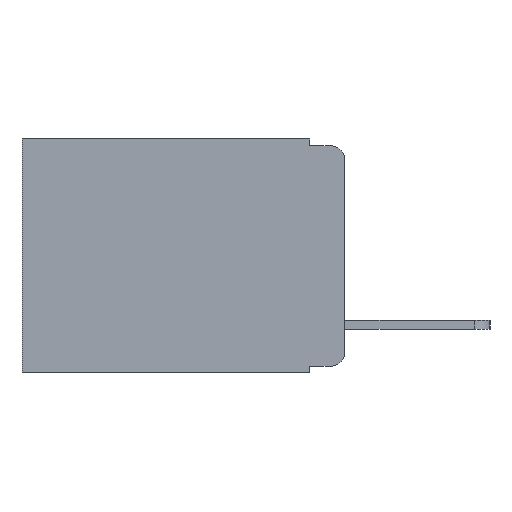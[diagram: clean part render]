
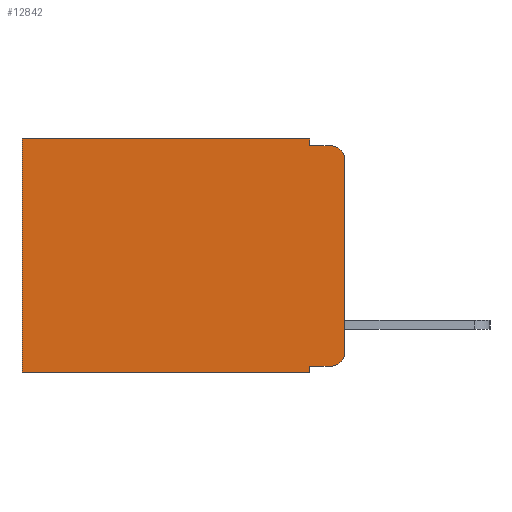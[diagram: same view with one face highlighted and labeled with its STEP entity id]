
A CAD part, left-side view. The second image highlights one B-rep face of the part: STEP entity #12842.
In plain terms, the highlighted planar face has unit normal (-1, 0, 0).
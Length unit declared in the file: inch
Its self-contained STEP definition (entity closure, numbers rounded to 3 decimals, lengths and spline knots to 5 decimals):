
#23 = CARTESIAN_POINT ( 'NONE',  ( 0.298, 0., -0.343 ) ) ;
#253 = FACE_OUTER_BOUND ( 'NONE', #6634, .T. ) ;
#566 = CARTESIAN_POINT ( 'NONE',  ( 0.298, 0.473, -0.343 ) ) ;
#773 = CARTESIAN_POINT ( 'NONE',  ( 0.298, 0., 0. ) ) ;
#2109 = DIRECTION ( 'NONE',  ( 0., 0., -1. ) ) ;
#2721 = DIRECTION ( 'NONE',  ( 0., 0., -1. ) ) ;
#2729 = VECTOR ( 'NONE', #3290, 39.37008 ) ;
#2751 = DIRECTION ( 'NONE',  ( 1., 0., 0. ) ) ;
#2919 = PLANE ( 'NONE',  #11009 ) ;
#2957 = EDGE_CURVE ( 'NONE', #6849, #13569, #20845, .T. ) ;
#3178 = ORIENTED_EDGE ( 'NONE', *, *, #3930, .F. ) ;
#3290 = DIRECTION ( 'NONE',  ( 0., 1., 0. ) ) ;
#3343 = EDGE_CURVE ( 'NONE', #10902, #22206, #21601, .T. ) ;
#3394 = CARTESIAN_POINT ( 'NONE',  ( 0.298, 0., 0. ) ) ;
#3669 = CARTESIAN_POINT ( 'NONE',  ( 0.298, 0.051, 0. ) ) ;
#3746 = DIRECTION ( 'NONE',  ( -1., 0., 0. ) ) ;
#3930 = EDGE_CURVE ( 'NONE', #8785, #4069, #19260, .T. ) ;
#3998 = EDGE_CURVE ( 'NONE', #8785, #4274, #18202, .T. ) ;
#4004 = EDGE_CURVE ( 'NONE', #4365, #4274, #5321, .T. ) ;
#4069 = VERTEX_POINT ( 'NONE', #11962 ) ;
#4159 = EDGE_CURVE ( 'NONE', #6849, #4365, #20669, .T. ) ;
#4177 = AXIS2_PLACEMENT_3D ( 'NONE', #6455, #3746, #4503 ) ;
#4274 = VERTEX_POINT ( 'NONE', #15161 ) ;
#4365 = VERTEX_POINT ( 'NONE', #20684 ) ;
#4404 = EDGE_CURVE ( 'NONE', #13569, #22206, #4499, .T. ) ;
#4458 = AXIS2_PLACEMENT_3D ( 'NONE', #13335, #13326, #20625 ) ;
#4499 = LINE ( 'NONE', #21514, #14571 ) ;
#4503 = DIRECTION ( 'NONE',  ( 0., 0., -1. ) ) ;
#4566 = EDGE_CURVE ( 'NONE', #13353, #10902, #12399, .T. ) ;
#4593 = EDGE_CURVE ( 'NONE', #13353, #18281, #21423, .T. ) ;
#4640 = EDGE_CURVE ( 'NONE', #18281, #4069, #10439, .T. ) ;
#5321 = LINE ( 'NONE', #13566, #22160 ) ;
#6455 = CARTESIAN_POINT ( 'NONE',  ( 0.298, 0.02, -0.313 ) ) ;
#6634 = EDGE_LOOP ( 'NONE', ( #3178, #12258, #16796, #21736, #22226, #18276, #18798, #11050, #15496, #20471 ) ) ;
#6849 = VERTEX_POINT ( 'NONE', #9258 ) ;
#7624 = CARTESIAN_POINT ( 'NONE',  ( 0.298, 0.02, -0.333 ) ) ;
#8089 = DIRECTION ( 'NONE',  ( 0., 1., 0. ) ) ;
#8785 = VERTEX_POINT ( 'NONE', #14760 ) ;
#8985 = CARTESIAN_POINT ( 'NONE',  ( 0.298, 0.051, -0.343 ) ) ;
#9171 = DIRECTION ( 'NONE',  ( 0., 0., -1. ) ) ;
#9258 = CARTESIAN_POINT ( 'NONE',  ( 0.298, 0.051, 0. ) ) ;
#10328 = CARTESIAN_POINT ( 'NONE',  ( 0.298, 0.473, 0. ) ) ;
#10439 = CIRCLE ( 'NONE', #4177, 0.02 ) ;
#10902 = VERTEX_POINT ( 'NONE', #8985 ) ;
#11009 = AXIS2_PLACEMENT_3D ( 'NONE', #3394, #2751, #2721 ) ;
#11050 = ORIENTED_EDGE ( 'NONE', *, *, #4566, .F. ) ;
#11850 = CARTESIAN_POINT ( 'NONE',  ( 0.298, 0., 0. ) ) ;
#11947 = DIRECTION ( 'NONE',  ( 0., 0., -1. ) ) ;
#11962 = CARTESIAN_POINT ( 'NONE',  ( 0.298, 0., -0.313 ) ) ;
#11963 = VECTOR ( 'NONE', #11977, 39.37008 ) ;
#11977 = DIRECTION ( 'NONE',  ( 0., -1., 0. ) ) ;
#12120 = DIRECTION ( 'NONE',  ( 0., 0., -1. ) ) ;
#12258 = ORIENTED_EDGE ( 'NONE', *, *, #3998, .T. ) ;
#12399 = LINE ( 'NONE', #19084, #16445 ) ;
#12842 = ADVANCED_FACE ( 'NONE', ( #253 ), #2919, .F. ) ;
#13326 = DIRECTION ( 'NONE',  ( -1., 0., 0. ) ) ;
#13335 = CARTESIAN_POINT ( 'NONE',  ( 0.298, 0.02, -0.03 ) ) ;
#13353 = VERTEX_POINT ( 'NONE', #15370 ) ;
#13379 = DIRECTION ( 'NONE',  ( 0., -1., 0. ) ) ;
#13566 = CARTESIAN_POINT ( 'NONE',  ( 0.298, 0.051, -0.01 ) ) ;
#13569 = VERTEX_POINT ( 'NONE', #10328 ) ;
#14571 = VECTOR ( 'NONE', #9171, 39.37008 ) ;
#14760 = CARTESIAN_POINT ( 'NONE',  ( 0.298, 0., -0.03 ) ) ;
#15161 = CARTESIAN_POINT ( 'NONE',  ( 0.298, 0.02, -0.01 ) ) ;
#15370 = CARTESIAN_POINT ( 'NONE',  ( 0.298, 0.051, -0.333 ) ) ;
#15429 = VECTOR ( 'NONE', #12120, 39.37008 ) ;
#15496 = ORIENTED_EDGE ( 'NONE', *, *, #4593, .T. ) ;
#15671 = VECTOR ( 'NONE', #2109, 39.37008 ) ;
#16120 = VECTOR ( 'NONE', #8089, 39.37008 ) ;
#16445 = VECTOR ( 'NONE', #11947, 39.37008 ) ;
#16796 = ORIENTED_EDGE ( 'NONE', *, *, #4004, .F. ) ;
#17062 = CARTESIAN_POINT ( 'NONE',  ( 0.298, 0.051, -0.333 ) ) ;
#18202 = CIRCLE ( 'NONE', #4458, 0.02 ) ;
#18276 = ORIENTED_EDGE ( 'NONE', *, *, #4404, .T. ) ;
#18281 = VERTEX_POINT ( 'NONE', #7624 ) ;
#18798 = ORIENTED_EDGE ( 'NONE', *, *, #3343, .F. ) ;
#19084 = CARTESIAN_POINT ( 'NONE',  ( 0.298, 0.051, 0. ) ) ;
#19260 = LINE ( 'NONE', #11850, #15429 ) ;
#20471 = ORIENTED_EDGE ( 'NONE', *, *, #4640, .T. ) ;
#20625 = DIRECTION ( 'NONE',  ( 0., 0., -1. ) ) ;
#20669 = LINE ( 'NONE', #3669, #15671 ) ;
#20684 = CARTESIAN_POINT ( 'NONE',  ( 0.298, 0.051, -0.01 ) ) ;
#20845 = LINE ( 'NONE', #773, #2729 ) ;
#21423 = LINE ( 'NONE', #17062, #11963 ) ;
#21514 = CARTESIAN_POINT ( 'NONE',  ( 0.298, 0.473, 0. ) ) ;
#21601 = LINE ( 'NONE', #23, #16120 ) ;
#21736 = ORIENTED_EDGE ( 'NONE', *, *, #4159, .F. ) ;
#22160 = VECTOR ( 'NONE', #13379, 39.37008 ) ;
#22206 = VERTEX_POINT ( 'NONE', #566 ) ;
#22226 = ORIENTED_EDGE ( 'NONE', *, *, #2957, .T. ) ;
